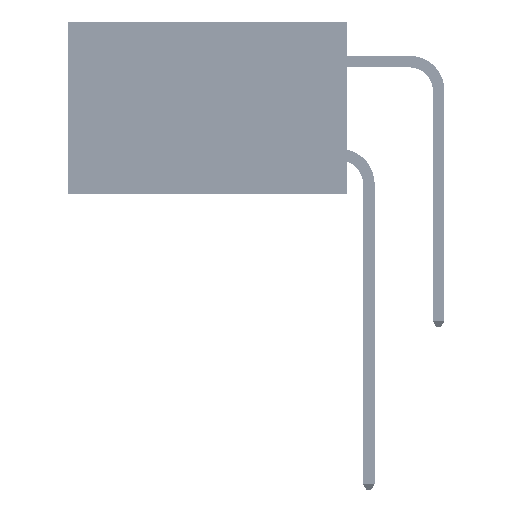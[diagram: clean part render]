
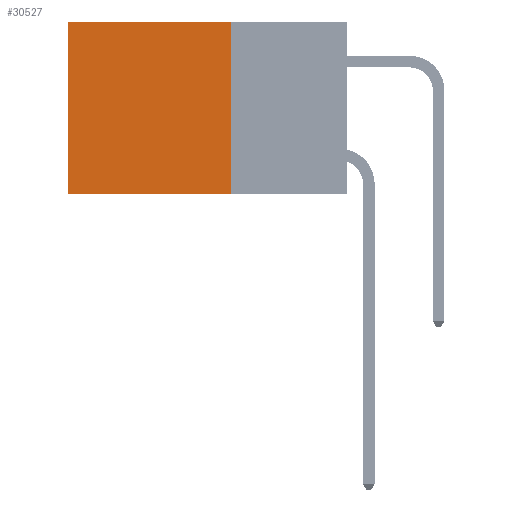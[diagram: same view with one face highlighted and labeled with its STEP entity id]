
A CAD part, left-side view. The second image highlights one B-rep face of the part: STEP entity #30527.
In plain terms, the highlighted planar face has unit normal (-1, 0, 0).
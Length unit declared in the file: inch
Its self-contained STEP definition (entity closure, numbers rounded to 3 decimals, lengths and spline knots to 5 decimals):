
#9405 = CARTESIAN_POINT ( 'NONE',  ( 0.2875, 0.6, 0. ) ) ;
#11846 = VECTOR ( 'NONE', #32944, 39.37008 ) ;
#11867 = ORIENTED_EDGE ( 'NONE', *, *, #48736, .F. ) ;
#15765 = LINE ( 'NONE', #28763, #11846 ) ;
#16337 = EDGE_CURVE ( 'NONE', #33927, #39095, #16645, .T. ) ;
#16346 = ORIENTED_EDGE ( 'NONE', *, *, #53953, .T. ) ;
#16645 = LINE ( 'NONE', #51456, #42118 ) ;
#17796 = ORIENTED_EDGE ( 'NONE', *, *, #45205, .T. ) ;
#18226 = VERTEX_POINT ( 'NONE', #43154 ) ;
#18563 = CARTESIAN_POINT ( 'NONE',  ( 0.2875, 0.25, 0. ) ) ;
#19279 = LINE ( 'NONE', #18563, #19956 ) ;
#19956 = VECTOR ( 'NONE', #26584, 39.37008 ) ;
#21050 = VECTOR ( 'NONE', #46458, 39.37008 ) ;
#22242 = PLANE ( 'NONE',  #31839 ) ;
#24966 = LINE ( 'NONE', #9405, #21050 ) ;
#26442 = DIRECTION ( 'NONE',  ( 1., 0., 0. ) ) ;
#26584 = DIRECTION ( 'NONE',  ( 0., 0., -1. ) ) ;
#26664 = FACE_OUTER_BOUND ( 'NONE', #46105, .T. ) ;
#28763 = CARTESIAN_POINT ( 'NONE',  ( 0.2875, 0.25, 0. ) ) ;
#30527 = ADVANCED_FACE ( 'NONE', ( #26664 ), #22242, .F. ) ;
#30993 = CARTESIAN_POINT ( 'NONE',  ( 0.2875, 0.25, 0. ) ) ;
#31763 = CARTESIAN_POINT ( 'NONE',  ( 0.2875, 0.25, -0.37 ) ) ;
#31839 = AXIS2_PLACEMENT_3D ( 'NONE', #30993, #26442, #35034 ) ;
#32944 = DIRECTION ( 'NONE',  ( 0., 1., 0. ) ) ;
#33927 = VERTEX_POINT ( 'NONE', #31763 ) ;
#35034 = DIRECTION ( 'NONE',  ( 0., 0., -1. ) ) ;
#38680 = CARTESIAN_POINT ( 'NONE',  ( 0.2875, 0.6, -0.37 ) ) ;
#39095 = VERTEX_POINT ( 'NONE', #38680 ) ;
#42118 = VECTOR ( 'NONE', #43026, 39.37008 ) ;
#42469 = VERTEX_POINT ( 'NONE', #43705 ) ;
#43026 = DIRECTION ( 'NONE',  ( 0., 1., 0. ) ) ;
#43154 = CARTESIAN_POINT ( 'NONE',  ( 0.2875, 0.6, 0. ) ) ;
#43705 = CARTESIAN_POINT ( 'NONE',  ( 0.2875, 0.25, 0. ) ) ;
#45205 = EDGE_CURVE ( 'NONE', #18226, #39095, #24966, .T. ) ;
#46105 = EDGE_LOOP ( 'NONE', ( #17796, #50999, #11867, #16346 ) ) ;
#46458 = DIRECTION ( 'NONE',  ( 0., 0., -1. ) ) ;
#48736 = EDGE_CURVE ( 'NONE', #42469, #33927, #19279, .T. ) ;
#50999 = ORIENTED_EDGE ( 'NONE', *, *, #16337, .F. ) ;
#51456 = CARTESIAN_POINT ( 'NONE',  ( 0.2875, 0.25, -0.37 ) ) ;
#53953 = EDGE_CURVE ( 'NONE', #42469, #18226, #15765, .T. ) ;
